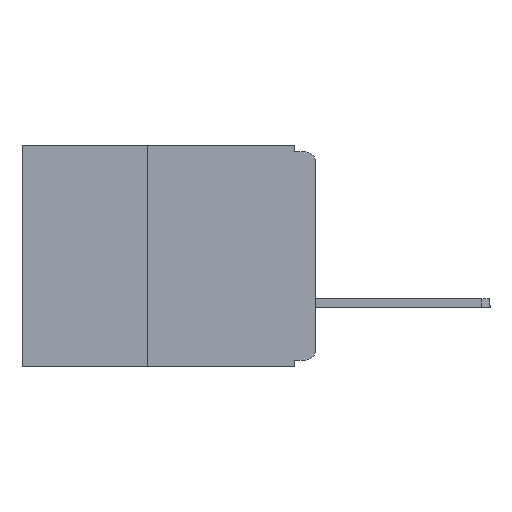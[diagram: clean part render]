
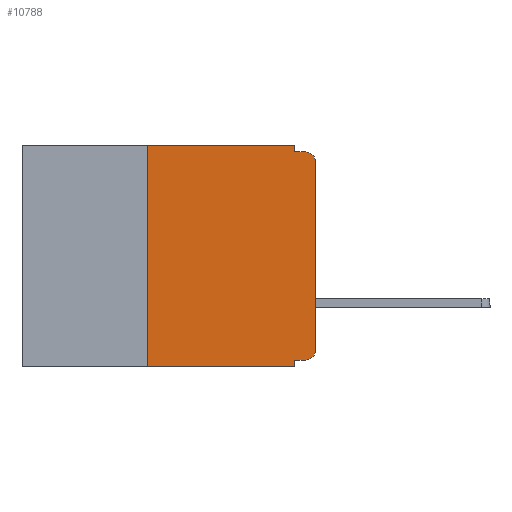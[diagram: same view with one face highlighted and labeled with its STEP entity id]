
A CAD part, left-side view. The second image highlights one B-rep face of the part: STEP entity #10788.
In plain terms, the highlighted planar face has unit normal (-1, 0, 0).
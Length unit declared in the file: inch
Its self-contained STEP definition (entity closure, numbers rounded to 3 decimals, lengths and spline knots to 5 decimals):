
#4 = CARTESIAN_POINT ( 'NONE',  ( 0., 0.25, 0. ) ) ;
#180 = CARTESIAN_POINT ( 'NONE',  ( 0., 0.031, -0.01 ) ) ;
#303 = CARTESIAN_POINT ( 'NONE',  ( 0., 0., 0. ) ) ;
#482 = CARTESIAN_POINT ( 'NONE',  ( 0., 0.437, 0. ) ) ;
#653 = VERTEX_POINT ( 'NONE', #4 ) ;
#709 = EDGE_CURVE ( 'NONE', #7144, #14382, #12442, .T. ) ;
#1597 = VECTOR ( 'NONE', #14298, 39.37008 ) ;
#1847 = DIRECTION ( 'NONE',  ( 1., 0., 0. ) ) ;
#1937 = EDGE_CURVE ( 'NONE', #653, #6778, #9082, .T. ) ;
#2082 = LINE ( 'NONE', #7618, #8571 ) ;
#2310 = CARTESIAN_POINT ( 'NONE',  ( 0., 0.031, 0. ) ) ;
#2371 = DIRECTION ( 'NONE',  ( 0., 0., -1. ) ) ;
#2977 = EDGE_CURVE ( 'NONE', #9439, #3692, #12773, .T. ) ;
#3076 = LINE ( 'NONE', #11846, #9528 ) ;
#3424 = DIRECTION ( 'NONE',  ( -1., 0., 0. ) ) ;
#3457 = VECTOR ( 'NONE', #11881, 39.37008 ) ;
#3610 = DIRECTION ( 'NONE',  ( 0., 0., -1. ) ) ;
#3692 = VERTEX_POINT ( 'NONE', #14346 ) ;
#3891 = LINE ( 'NONE', #8597, #13352 ) ;
#3934 = CARTESIAN_POINT ( 'NONE',  ( 0., 0., -0.305 ) ) ;
#4248 = VERTEX_POINT ( 'NONE', #13466 ) ;
#4353 = ORIENTED_EDGE ( 'NONE', *, *, #4692, .T. ) ;
#4692 = EDGE_CURVE ( 'NONE', #12757, #7574, #2082, .T. ) ;
#4698 = LINE ( 'NONE', #7105, #1597 ) ;
#6146 = ORIENTED_EDGE ( 'NONE', *, *, #13731, .F. ) ;
#6386 = ORIENTED_EDGE ( 'NONE', *, *, #14539, .F. ) ;
#6778 = VERTEX_POINT ( 'NONE', #15860 ) ;
#6959 = PLANE ( 'NONE',  #8798 ) ;
#6963 = ORIENTED_EDGE ( 'NONE', *, *, #14857, .F. ) ;
#6981 = CARTESIAN_POINT ( 'NONE',  ( 0., 0.015, -0.305 ) ) ;
#7105 = CARTESIAN_POINT ( 'NONE',  ( 0., 0., -0.32 ) ) ;
#7144 = VERTEX_POINT ( 'NONE', #10324 ) ;
#7574 = VERTEX_POINT ( 'NONE', #7902 ) ;
#7600 = DIRECTION ( 'NONE',  ( 0., -1., 0. ) ) ;
#7618 = CARTESIAN_POINT ( 'NONE',  ( 0., 0.437, -0.33 ) ) ;
#7827 = VERTEX_POINT ( 'NONE', #180 ) ;
#7902 = CARTESIAN_POINT ( 'NONE',  ( 0., 0.031, -0.33 ) ) ;
#8016 = ORIENTED_EDGE ( 'NONE', *, *, #11723, .F. ) ;
#8040 = ORIENTED_EDGE ( 'NONE', *, *, #2977, .T. ) ;
#8245 = ORIENTED_EDGE ( 'NONE', *, *, #1937, .F. ) ;
#8383 = LINE ( 'NONE', #303, #14302 ) ;
#8571 = VECTOR ( 'NONE', #7600, 39.37008 ) ;
#8597 = CARTESIAN_POINT ( 'NONE',  ( 0., 0.031, -0.33 ) ) ;
#8751 = EDGE_CURVE ( 'NONE', #14382, #9439, #8383, .T. ) ;
#8798 = AXIS2_PLACEMENT_3D ( 'NONE', #482, #1847, #10806 ) ;
#8921 = FACE_OUTER_BOUND ( 'NONE', #15267, .T. ) ;
#9044 = ORIENTED_EDGE ( 'NONE', *, *, #10842, .F. ) ;
#9068 = ORIENTED_EDGE ( 'NONE', *, *, #8751, .T. ) ;
#9082 = LINE ( 'NONE', #15405, #12232 ) ;
#9439 = VERTEX_POINT ( 'NONE', #9482 ) ;
#9482 = CARTESIAN_POINT ( 'NONE',  ( 0., 0., -0.025 ) ) ;
#9497 = CARTESIAN_POINT ( 'NONE',  ( 0., 0., -0.01 ) ) ;
#9528 = VECTOR ( 'NONE', #14139, 39.37008 ) ;
#9876 = DIRECTION ( 'NONE',  ( 0., 0., -1. ) ) ;
#10284 = LINE ( 'NONE', #9497, #3457 ) ;
#10324 = CARTESIAN_POINT ( 'NONE',  ( 0., 0.015, -0.32 ) ) ;
#10788 = ADVANCED_FACE ( 'NONE', ( #8921 ), #6959, .F. ) ;
#10806 = DIRECTION ( 'NONE',  ( 0., 0., -1. ) ) ;
#10842 = EDGE_CURVE ( 'NONE', #7144, #4248, #4698, .T. ) ;
#10869 = AXIS2_PLACEMENT_3D ( 'NONE', #13257, #13229, #13223 ) ;
#11723 = EDGE_CURVE ( 'NONE', #4248, #7574, #3891, .T. ) ;
#11846 = CARTESIAN_POINT ( 'NONE',  ( 0., 0.25, -0.33 ) ) ;
#11881 = DIRECTION ( 'NONE',  ( 0., -1., 0. ) ) ;
#12114 = VECTOR ( 'NONE', #3610, 39.37008 ) ;
#12232 = VECTOR ( 'NONE', #15648, 39.37008 ) ;
#12442 = CIRCLE ( 'NONE', #15441, 0.015 ) ;
#12575 = CARTESIAN_POINT ( 'NONE',  ( 0., 0.25, -0.33 ) ) ;
#12757 = VERTEX_POINT ( 'NONE', #12575 ) ;
#12773 = CIRCLE ( 'NONE', #10869, 0.015 ) ;
#13223 = DIRECTION ( 'NONE',  ( 0., 0., -1. ) ) ;
#13229 = DIRECTION ( 'NONE',  ( -1., 0., 0. ) ) ;
#13257 = CARTESIAN_POINT ( 'NONE',  ( 0., 0.015, -0.025 ) ) ;
#13352 = VECTOR ( 'NONE', #9876, 39.37008 ) ;
#13466 = CARTESIAN_POINT ( 'NONE',  ( 0., 0.031, -0.32 ) ) ;
#13731 = EDGE_CURVE ( 'NONE', #12757, #653, #3076, .T. ) ;
#14072 = DIRECTION ( 'NONE',  ( 0., 0., 1. ) ) ;
#14139 = DIRECTION ( 'NONE',  ( 0., 0., 1. ) ) ;
#14298 = DIRECTION ( 'NONE',  ( 0., 1., 0. ) ) ;
#14302 = VECTOR ( 'NONE', #14072, 39.37008 ) ;
#14346 = CARTESIAN_POINT ( 'NONE',  ( 0., 0.015, -0.01 ) ) ;
#14382 = VERTEX_POINT ( 'NONE', #3934 ) ;
#14539 = EDGE_CURVE ( 'NONE', #7827, #3692, #10284, .T. ) ;
#14803 = ORIENTED_EDGE ( 'NONE', *, *, #709, .T. ) ;
#14857 = EDGE_CURVE ( 'NONE', #6778, #7827, #15821, .T. ) ;
#15267 = EDGE_LOOP ( 'NONE', ( #9068, #8040, #6386, #6963, #8245, #6146, #4353, #8016, #9044, #14803 ) ) ;
#15405 = CARTESIAN_POINT ( 'NONE',  ( 0., 0.437, 0. ) ) ;
#15441 = AXIS2_PLACEMENT_3D ( 'NONE', #6981, #3424, #2371 ) ;
#15648 = DIRECTION ( 'NONE',  ( 0., -1., 0. ) ) ;
#15821 = LINE ( 'NONE', #2310, #12114 ) ;
#15860 = CARTESIAN_POINT ( 'NONE',  ( 0., 0.031, 0. ) ) ;
